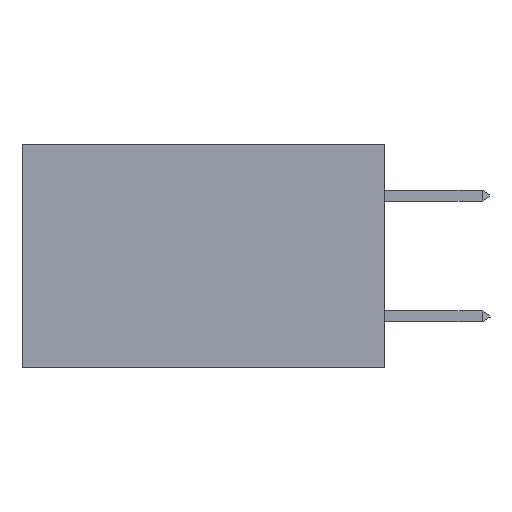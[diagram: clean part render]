
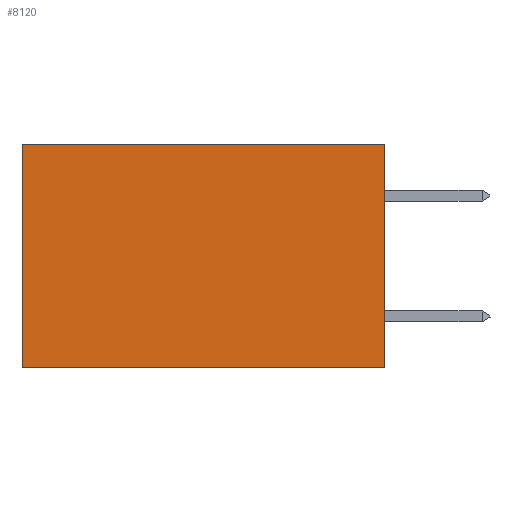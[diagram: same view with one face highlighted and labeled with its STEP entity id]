
A CAD part, left-side view. The second image highlights one B-rep face of the part: STEP entity #8120.
In plain terms, the highlighted planar face has unit normal (-1, 0, 0).
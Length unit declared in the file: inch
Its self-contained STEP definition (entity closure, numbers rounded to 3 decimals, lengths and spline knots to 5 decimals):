
#12 = LINE ( 'NONE', #1843, #3427 ) ;
#36 = ORIENTED_EDGE ( 'NONE', *, *, #2067, .F. ) ;
#206 = DIRECTION ( 'NONE',  ( 1., 0., 0. ) ) ;
#545 = EDGE_CURVE ( 'NONE', #4681, #4635, #6701, .T. ) ;
#1044 = LINE ( 'NONE', #5055, #4045 ) ;
#1066 = VERTEX_POINT ( 'NONE', #3098 ) ;
#1368 = CARTESIAN_POINT ( 'NONE',  ( 0.2875, 0.6, 0. ) ) ;
#1707 = DIRECTION ( 'NONE',  ( 0., 1., 0. ) ) ;
#1843 = CARTESIAN_POINT ( 'NONE',  ( 0.2875, 0., 0. ) ) ;
#2067 = EDGE_CURVE ( 'NONE', #4058, #4635, #1044, .T. ) ;
#2350 = VECTOR ( 'NONE', #2517, 39.37008 ) ;
#2452 = DIRECTION ( 'NONE',  ( 0., 1., 0. ) ) ;
#2482 = ORIENTED_EDGE ( 'NONE', *, *, #6618, .F. ) ;
#2517 = DIRECTION ( 'NONE',  ( 0., 0., -1. ) ) ;
#2816 = AXIS2_PLACEMENT_3D ( 'NONE', #7679, #206, #5676 ) ;
#3098 = CARTESIAN_POINT ( 'NONE',  ( 0.2875, 0., 0. ) ) ;
#3405 = FACE_OUTER_BOUND ( 'NONE', #7566, .T. ) ;
#3427 = VECTOR ( 'NONE', #2452, 39.37008 ) ;
#3656 = ORIENTED_EDGE ( 'NONE', *, *, #545, .T. ) ;
#4045 = VECTOR ( 'NONE', #1707, 39.37008 ) ;
#4058 = VERTEX_POINT ( 'NONE', #5960 ) ;
#4275 = CARTESIAN_POINT ( 'NONE',  ( 0.2875, 0., 0. ) ) ;
#4353 = ORIENTED_EDGE ( 'NONE', *, *, #7687, .T. ) ;
#4635 = VERTEX_POINT ( 'NONE', #8540 ) ;
#4681 = VERTEX_POINT ( 'NONE', #1368 ) ;
#5055 = CARTESIAN_POINT ( 'NONE',  ( 0.2875, 0., -0.37 ) ) ;
#5676 = DIRECTION ( 'NONE',  ( 0., 0., -1. ) ) ;
#5683 = LINE ( 'NONE', #4275, #8106 ) ;
#5960 = CARTESIAN_POINT ( 'NONE',  ( 0.2875, 0., -0.37 ) ) ;
#6330 = DIRECTION ( 'NONE',  ( 0., 0., -1. ) ) ;
#6578 = CARTESIAN_POINT ( 'NONE',  ( 0.2875, 0.6, 0. ) ) ;
#6618 = EDGE_CURVE ( 'NONE', #1066, #4058, #5683, .T. ) ;
#6701 = LINE ( 'NONE', #6578, #2350 ) ;
#7566 = EDGE_LOOP ( 'NONE', ( #3656, #36, #2482, #4353 ) ) ;
#7606 = PLANE ( 'NONE',  #2816 ) ;
#7679 = CARTESIAN_POINT ( 'NONE',  ( 0.2875, 0., 0. ) ) ;
#7687 = EDGE_CURVE ( 'NONE', #1066, #4681, #12, .T. ) ;
#8106 = VECTOR ( 'NONE', #6330, 39.37008 ) ;
#8120 = ADVANCED_FACE ( 'NONE', ( #3405 ), #7606, .F. ) ;
#8540 = CARTESIAN_POINT ( 'NONE',  ( 0.2875, 0.6, -0.37 ) ) ;
